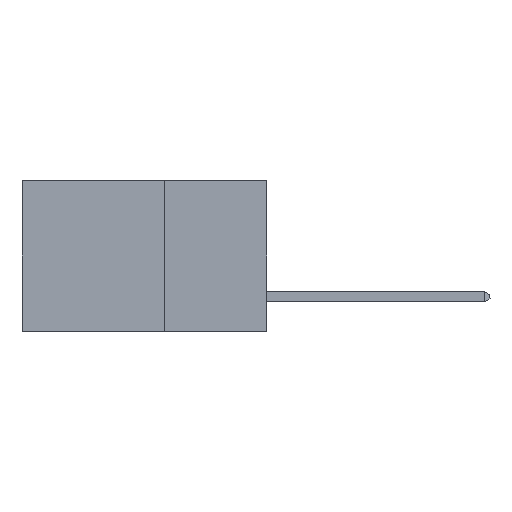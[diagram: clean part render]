
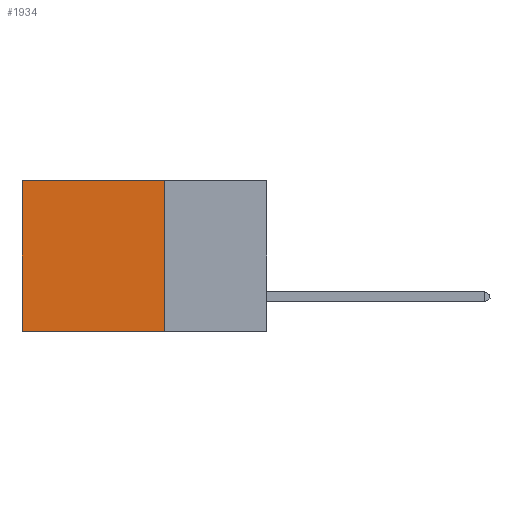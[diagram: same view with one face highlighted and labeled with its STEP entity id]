
A CAD part, left-side view. The second image highlights one B-rep face of the part: STEP entity #1934.
In plain terms, the highlighted planar face has unit normal (-1, 0, 0).
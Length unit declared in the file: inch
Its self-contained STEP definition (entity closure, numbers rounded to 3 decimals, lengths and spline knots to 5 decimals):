
#252 = ORIENTED_EDGE ( 'NONE', *, *, #3191, .F. ) ;
#280 = VERTEX_POINT ( 'NONE', #7858 ) ;
#801 = CARTESIAN_POINT ( 'NONE',  ( 0.2875, 0.25, 0. ) ) ;
#1126 = EDGE_CURVE ( 'NONE', #3582, #12224, #5647, .T. ) ;
#1271 = FACE_OUTER_BOUND ( 'NONE', #10583, .T. ) ;
#1934 = ADVANCED_FACE ( 'NONE', ( #1271 ), #3385, .F. ) ;
#1961 = CARTESIAN_POINT ( 'NONE',  ( 0.2875, 0.25, -0.37 ) ) ;
#2041 = DIRECTION ( 'NONE',  ( 0., 1., 0. ) ) ;
#2184 = LINE ( 'NONE', #10036, #4220 ) ;
#3035 = VECTOR ( 'NONE', #8066, 39.37008 ) ;
#3132 = ORIENTED_EDGE ( 'NONE', *, *, #5532, .T. ) ;
#3191 = EDGE_CURVE ( 'NONE', #3582, #11263, #2184, .T. ) ;
#3384 = DIRECTION ( 'NONE',  ( 0., 0., -1. ) ) ;
#3385 = PLANE ( 'NONE',  #6760 ) ;
#3582 = VERTEX_POINT ( 'NONE', #6212 ) ;
#3932 = CARTESIAN_POINT ( 'NONE',  ( 0.2875, 0.25, -0.37 ) ) ;
#4220 = VECTOR ( 'NONE', #3384, 39.37008 ) ;
#5238 = ORIENTED_EDGE ( 'NONE', *, *, #1126, .T. ) ;
#5532 = EDGE_CURVE ( 'NONE', #12224, #280, #8359, .T. ) ;
#5647 = LINE ( 'NONE', #801, #3035 ) ;
#5790 = LINE ( 'NONE', #1961, #7789 ) ;
#6015 = VECTOR ( 'NONE', #7837, 39.37008 ) ;
#6212 = CARTESIAN_POINT ( 'NONE',  ( 0.2875, 0.25, 0. ) ) ;
#6399 = ORIENTED_EDGE ( 'NONE', *, *, #9023, .F. ) ;
#6760 = AXIS2_PLACEMENT_3D ( 'NONE', #9526, #11472, #12005 ) ;
#7789 = VECTOR ( 'NONE', #2041, 39.37008 ) ;
#7814 = CARTESIAN_POINT ( 'NONE',  ( 0.2875, 0.6, 0. ) ) ;
#7837 = DIRECTION ( 'NONE',  ( 0., 0., -1. ) ) ;
#7858 = CARTESIAN_POINT ( 'NONE',  ( 0.2875, 0.6, -0.37 ) ) ;
#8066 = DIRECTION ( 'NONE',  ( 0., 1., 0. ) ) ;
#8359 = LINE ( 'NONE', #7814, #6015 ) ;
#9023 = EDGE_CURVE ( 'NONE', #11263, #280, #5790, .T. ) ;
#9526 = CARTESIAN_POINT ( 'NONE',  ( 0.2875, 0.25, 0. ) ) ;
#10036 = CARTESIAN_POINT ( 'NONE',  ( 0.2875, 0.25, 0. ) ) ;
#10397 = CARTESIAN_POINT ( 'NONE',  ( 0.2875, 0.6, 0. ) ) ;
#10583 = EDGE_LOOP ( 'NONE', ( #3132, #6399, #252, #5238 ) ) ;
#11263 = VERTEX_POINT ( 'NONE', #3932 ) ;
#11472 = DIRECTION ( 'NONE',  ( 1., 0., 0. ) ) ;
#12005 = DIRECTION ( 'NONE',  ( 0., 0., -1. ) ) ;
#12224 = VERTEX_POINT ( 'NONE', #10397 ) ;
